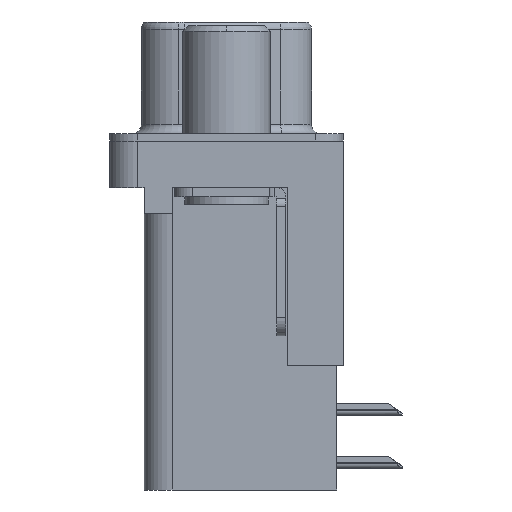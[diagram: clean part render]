
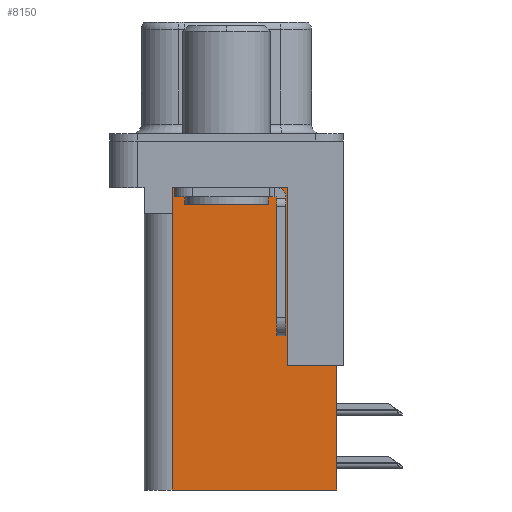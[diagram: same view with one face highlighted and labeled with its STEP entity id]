
A CAD part, left-side view. The second image highlights one B-rep face of the part: STEP entity #8150.
In plain terms, the highlighted planar face has unit normal (-1, 0, 0).
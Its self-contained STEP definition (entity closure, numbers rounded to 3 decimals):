
#94 = CARTESIAN_POINT ( 'NONE',  ( 3.7, 2.895, -3.9 ) ) ;
#757 = VECTOR ( 'NONE', #11542, 1000. ) ;
#777 = CARTESIAN_POINT ( 'NONE',  ( 3.7, -3.295, -18.76 ) ) ;
#2516 = CARTESIAN_POINT ( 'NONE',  ( 3.7, -3.295, -2.5 ) ) ;
#2742 = LINE ( 'NONE', #2842, #6778 ) ;
#2842 = CARTESIAN_POINT ( 'NONE',  ( 3.7, -3.295, -18.76 ) ) ;
#2959 = ORIENTED_EDGE ( 'NONE', *, *, #9357, .T. ) ;
#3520 = LINE ( 'NONE', #14203, #16362 ) ;
#3621 = ORIENTED_EDGE ( 'NONE', *, *, #9865, .F. ) ;
#3852 = CARTESIAN_POINT ( 'NONE',  ( 3.7, 2.925, -3.9 ) ) ;
#4051 = LINE ( 'NONE', #22829, #13296 ) ;
#4180 = DIRECTION ( 'NONE',  ( 0., 0., 1. ) ) ;
#4274 = DIRECTION ( 'NONE',  ( 1., 0., 0. ) ) ;
#5842 = ORIENTED_EDGE ( 'NONE', *, *, #21586, .F. ) ;
#5878 = EDGE_CURVE ( 'NONE', #8810, #21465, #3520, .T. ) ;
#6313 = EDGE_CURVE ( 'NONE', #15135, #8355, #4051, .T. ) ;
#6778 = VECTOR ( 'NONE', #18649, 1000. ) ;
#7648 = VERTEX_POINT ( 'NONE', #16142 ) ;
#8130 = FACE_OUTER_BOUND ( 'NONE', #10356, .T. ) ;
#8150 = ADVANCED_FACE ( 'NONE', ( #8130 ), #20080, .F. ) ;
#8355 = VERTEX_POINT ( 'NONE', #15256 ) ;
#8468 = DIRECTION ( 'NONE',  ( 0., 1., 0. ) ) ;
#8810 = VERTEX_POINT ( 'NONE', #17226 ) ;
#9357 = EDGE_CURVE ( 'NONE', #10678, #18163, #14651, .T. ) ;
#9847 = LINE ( 'NONE', #10879, #14508 ) ;
#9865 = EDGE_CURVE ( 'NONE', #17079, #18163, #13515, .T. ) ;
#10349 = EDGE_CURVE ( 'NONE', #8355, #10678, #13495, .T. ) ;
#10356 = EDGE_LOOP ( 'NONE', ( #15896, #14659, #2959, #3621, #5842, #15863, #16555, #17782 ) ) ;
#10678 = VERTEX_POINT ( 'NONE', #94 ) ;
#10879 = CARTESIAN_POINT ( 'NONE',  ( 3.7, -3.295, -18.76 ) ) ;
#11542 = DIRECTION ( 'NONE',  ( 0., 1., 0. ) ) ;
#11894 = CARTESIAN_POINT ( 'NONE',  ( 3.7, -6.295, -12.05 ) ) ;
#12033 = CARTESIAN_POINT ( 'NONE',  ( 3.7, 2.925, -18.76 ) ) ;
#12579 = EDGE_CURVE ( 'NONE', #8810, #7648, #20431, .T. ) ;
#13296 = VECTOR ( 'NONE', #17636, 1000. ) ;
#13495 = LINE ( 'NONE', #19871, #22491 ) ;
#13515 = LINE ( 'NONE', #21746, #21933 ) ;
#14203 = CARTESIAN_POINT ( 'NONE',  ( 3.7, -5.925, -2. ) ) ;
#14508 = VECTOR ( 'NONE', #18044, 1000. ) ;
#14651 = LINE ( 'NONE', #22256, #757 ) ;
#14659 = ORIENTED_EDGE ( 'NONE', *, *, #10349, .T. ) ;
#15135 = VERTEX_POINT ( 'NONE', #2516 ) ;
#15256 = CARTESIAN_POINT ( 'NONE',  ( 3.7, 2.895, -2.5 ) ) ;
#15613 = VECTOR ( 'NONE', #8468, 1000. ) ;
#15863 = ORIENTED_EDGE ( 'NONE', *, *, #5878, .F. ) ;
#15896 = ORIENTED_EDGE ( 'NONE', *, *, #6313, .T. ) ;
#15997 = DIRECTION ( 'NONE',  ( 0., 0., -1. ) ) ;
#16142 = CARTESIAN_POINT ( 'NONE',  ( 3.7, -3.295, -12.05 ) ) ;
#16209 = DIRECTION ( 'NONE',  ( 0., 0., -1. ) ) ;
#16274 = EDGE_CURVE ( 'NONE', #7648, #15135, #2742, .T. ) ;
#16362 = VECTOR ( 'NONE', #15997, 1000. ) ;
#16505 = DIRECTION ( 'NONE',  ( 0., 1., 0. ) ) ;
#16555 = ORIENTED_EDGE ( 'NONE', *, *, #12579, .T. ) ;
#17079 = VERTEX_POINT ( 'NONE', #12033 ) ;
#17226 = CARTESIAN_POINT ( 'NONE',  ( 3.7, -5.925, -12.05 ) ) ;
#17254 = AXIS2_PLACEMENT_3D ( 'NONE', #777, #4274, #16505 ) ;
#17636 = DIRECTION ( 'NONE',  ( 0., 1., 0. ) ) ;
#17782 = ORIENTED_EDGE ( 'NONE', *, *, #16274, .T. ) ;
#18044 = DIRECTION ( 'NONE',  ( 0., 1., 0. ) ) ;
#18163 = VERTEX_POINT ( 'NONE', #3852 ) ;
#18649 = DIRECTION ( 'NONE',  ( 0., 0., 1. ) ) ;
#19406 = CARTESIAN_POINT ( 'NONE',  ( 3.7, -5.925, -18.76 ) ) ;
#19871 = CARTESIAN_POINT ( 'NONE',  ( 3.7, 2.895, -3.9 ) ) ;
#20080 = PLANE ( 'NONE',  #17254 ) ;
#20431 = LINE ( 'NONE', #11894, #15613 ) ;
#21465 = VERTEX_POINT ( 'NONE', #19406 ) ;
#21586 = EDGE_CURVE ( 'NONE', #21465, #17079, #9847, .T. ) ;
#21746 = CARTESIAN_POINT ( 'NONE',  ( 3.7, 2.925, -18.76 ) ) ;
#21933 = VECTOR ( 'NONE', #4180, 1000. ) ;
#22256 = CARTESIAN_POINT ( 'NONE',  ( 3.7, 0., -3.9 ) ) ;
#22491 = VECTOR ( 'NONE', #16209, 1000. ) ;
#22829 = CARTESIAN_POINT ( 'NONE',  ( 3.7, -3.295, -2.5 ) ) ;
